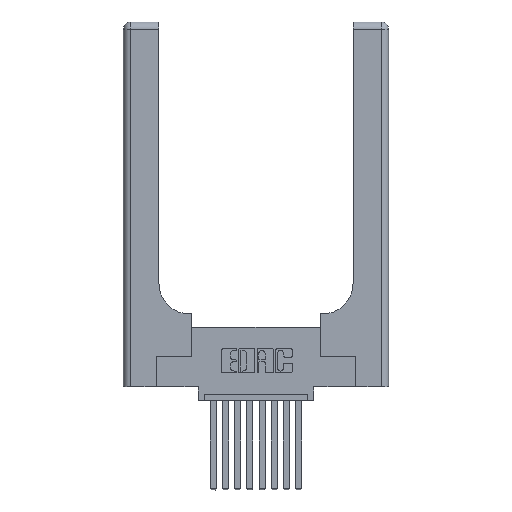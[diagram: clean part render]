
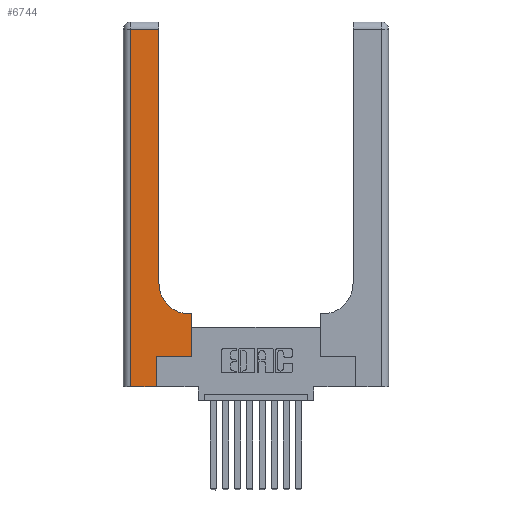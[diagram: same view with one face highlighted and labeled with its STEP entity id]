
A CAD part, top view. The second image highlights one B-rep face of the part: STEP entity #6744.
In plain terms, the highlighted planar face has unit normal (0, 0, 1).
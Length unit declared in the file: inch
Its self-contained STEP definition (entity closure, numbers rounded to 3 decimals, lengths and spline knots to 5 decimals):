
#504 = CARTESIAN_POINT ( 'NONE',  ( 0.2915, 0.85, 0.37 ) ) ;
#707 = EDGE_CURVE ( 'NONE', #6884, #8948, #5381, .T. ) ;
#745 = CARTESIAN_POINT ( 'NONE',  ( 0.269, 0., 0.37 ) ) ;
#1484 = LINE ( 'NONE', #9930, #14986 ) ;
#2545 = ORIENTED_EDGE ( 'NONE', *, *, #707, .T. ) ;
#2745 = DIRECTION ( 'NONE',  ( 0., 0., -1. ) ) ;
#2805 = AXIS2_PLACEMENT_3D ( 'NONE', #13094, #8203, #13288 ) ;
#2919 = ORIENTED_EDGE ( 'NONE', *, *, #3807, .T. ) ;
#3124 = DIRECTION ( 'NONE',  ( 0., 1., 0. ) ) ;
#3141 = ORIENTED_EDGE ( 'NONE', *, *, #14019, .T. ) ;
#3279 = FACE_OUTER_BOUND ( 'NONE', #11171, .T. ) ;
#3395 = LINE ( 'NONE', #10300, #4151 ) ;
#3453 = EDGE_CURVE ( 'NONE', #3822, #9282, #8347, .T. ) ;
#3807 = EDGE_CURVE ( 'NONE', #8232, #5486, #1484, .T. ) ;
#3822 = VERTEX_POINT ( 'NONE', #504 ) ;
#3823 = DIRECTION ( 'NONE',  ( 1., 0., 0. ) ) ;
#3824 = CARTESIAN_POINT ( 'NONE',  ( 0.5585, 0.25, 0.37 ) ) ;
#3834 = VECTOR ( 'NONE', #3823, 39.37008 ) ;
#3982 = VERTEX_POINT ( 'NONE', #8047 ) ;
#4027 = DIRECTION ( 'NONE',  ( 1., 0., 0. ) ) ;
#4079 = ORIENTED_EDGE ( 'NONE', *, *, #7169, .T. ) ;
#4151 = VECTOR ( 'NONE', #6782, 39.37008 ) ;
#5365 = EDGE_CURVE ( 'NONE', #8948, #3982, #15152, .T. ) ;
#5381 = LINE ( 'NONE', #3824, #11224 ) ;
#5486 = VERTEX_POINT ( 'NONE', #15219 ) ;
#5742 = LINE ( 'NONE', #14605, #3834 ) ;
#5839 = VECTOR ( 'NONE', #10975, 39.37008 ) ;
#6021 = DIRECTION ( 'NONE',  ( 1., 0., 0. ) ) ;
#6035 = CARTESIAN_POINT ( 'NONE',  ( 0.269, 0., 0.37 ) ) ;
#6108 = CARTESIAN_POINT ( 'NONE',  ( 0.2915, 0.6, 0.37 ) ) ;
#6216 = CARTESIAN_POINT ( 'NONE',  ( 0.5585, 0.25, 0.37 ) ) ;
#6361 = AXIS2_PLACEMENT_3D ( 'NONE', #7449, #2745, #4027 ) ;
#6482 = EDGE_CURVE ( 'NONE', #13893, #11865, #12765, .T. ) ;
#6744 = ADVANCED_FACE ( 'NONE', ( #3279 ), #15603, .F. ) ;
#6782 = DIRECTION ( 'NONE',  ( -1., 0., 0. ) ) ;
#6884 = VERTEX_POINT ( 'NONE', #6216 ) ;
#7169 = EDGE_CURVE ( 'NONE', #5486, #13893, #5742, .T. ) ;
#7434 = ORIENTED_EDGE ( 'NONE', *, *, #14416, .T. ) ;
#7449 = CARTESIAN_POINT ( 'NONE',  ( 0.5415, 0.85, 0.37 ) ) ;
#7519 = DIRECTION ( 'NONE',  ( 0., 1., 0. ) ) ;
#7946 = ORIENTED_EDGE ( 'NONE', *, *, #9344, .T. ) ;
#8047 = CARTESIAN_POINT ( 'NONE',  ( 0.5415, 0.6, 0.37 ) ) ;
#8203 = DIRECTION ( 'NONE',  ( 0., 0., -1. ) ) ;
#8232 = VERTEX_POINT ( 'NONE', #13679 ) ;
#8347 = LINE ( 'NONE', #13335, #12498 ) ;
#8948 = VERTEX_POINT ( 'NONE', #15371 ) ;
#9282 = VERTEX_POINT ( 'NONE', #15250 ) ;
#9344 = EDGE_CURVE ( 'NONE', #9282, #8232, #3395, .T. ) ;
#9545 = ORIENTED_EDGE ( 'NONE', *, *, #5365, .T. ) ;
#9546 = VECTOR ( 'NONE', #3124, 39.37008 ) ;
#9632 = DIRECTION ( 'NONE',  ( 0., 1., 0. ) ) ;
#9930 = CARTESIAN_POINT ( 'NONE',  ( 0.06, 3., 0.37 ) ) ;
#10083 = DIRECTION ( 'NONE',  ( 0., -1., 0. ) ) ;
#10300 = CARTESIAN_POINT ( 'NONE',  ( 0., 2.94, 0.37 ) ) ;
#10309 = ORIENTED_EDGE ( 'NONE', *, *, #3453, .T. ) ;
#10353 = VECTOR ( 'NONE', #6021, 39.37008 ) ;
#10875 = CARTESIAN_POINT ( 'NONE',  ( 0.269, 0.25, 0.37 ) ) ;
#10975 = DIRECTION ( 'NONE',  ( -1., 0., 0. ) ) ;
#11171 = EDGE_LOOP ( 'NONE', ( #10309, #7946, #2919, #4079, #15535, #7434, #2545, #9545, #3141 ) ) ;
#11224 = VECTOR ( 'NONE', #7519, 39.37008 ) ;
#11865 = VERTEX_POINT ( 'NONE', #15154 ) ;
#12498 = VECTOR ( 'NONE', #9632, 39.37008 ) ;
#12765 = LINE ( 'NONE', #745, #9546 ) ;
#13017 = CIRCLE ( 'NONE', #6361, 0.25 ) ;
#13094 = CARTESIAN_POINT ( 'NONE',  ( 0., 3., 0.37 ) ) ;
#13288 = DIRECTION ( 'NONE',  ( -1., 0., 0. ) ) ;
#13335 = CARTESIAN_POINT ( 'NONE',  ( 0.2915, 3., 0.37 ) ) ;
#13679 = CARTESIAN_POINT ( 'NONE',  ( 0.06, 2.94, 0.37 ) ) ;
#13893 = VERTEX_POINT ( 'NONE', #6035 ) ;
#14019 = EDGE_CURVE ( 'NONE', #3982, #3822, #13017, .T. ) ;
#14416 = EDGE_CURVE ( 'NONE', #11865, #6884, #14530, .T. ) ;
#14530 = LINE ( 'NONE', #10875, #10353 ) ;
#14605 = CARTESIAN_POINT ( 'NONE',  ( 0., 0., 0.37 ) ) ;
#14986 = VECTOR ( 'NONE', #10083, 39.37008 ) ;
#15152 = LINE ( 'NONE', #6108, #5839 ) ;
#15154 = CARTESIAN_POINT ( 'NONE',  ( 0.269, 0.25, 0.37 ) ) ;
#15219 = CARTESIAN_POINT ( 'NONE',  ( 0.06, 0., 0.37 ) ) ;
#15250 = CARTESIAN_POINT ( 'NONE',  ( 0.2915, 2.94, 0.37 ) ) ;
#15371 = CARTESIAN_POINT ( 'NONE',  ( 0.5585, 0.6, 0.37 ) ) ;
#15535 = ORIENTED_EDGE ( 'NONE', *, *, #6482, .T. ) ;
#15603 = PLANE ( 'NONE',  #2805 ) ;
